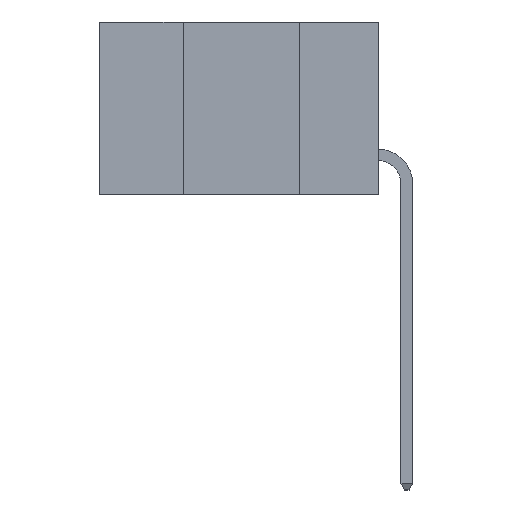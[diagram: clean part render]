
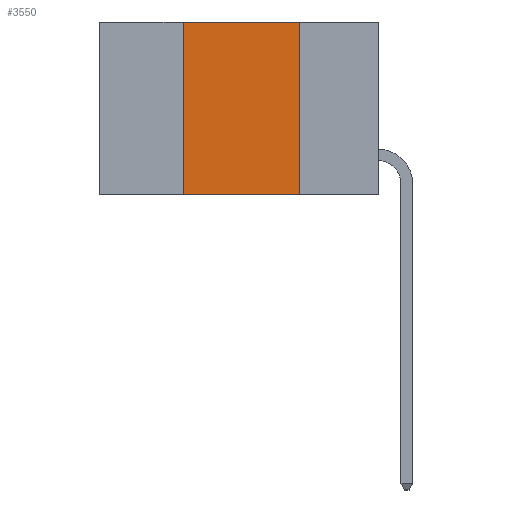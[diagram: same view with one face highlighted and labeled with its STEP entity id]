
A CAD part, left-side view. The second image highlights one B-rep face of the part: STEP entity #3550.
In plain terms, the highlighted planar face has unit normal (-1, 0, 0).
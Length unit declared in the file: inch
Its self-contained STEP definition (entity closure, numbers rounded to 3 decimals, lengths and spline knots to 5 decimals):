
#623 = AXIS2_PLACEMENT_3D ( 'NONE', #3833, #1502, #4617 ) ;
#794 = CARTESIAN_POINT ( 'NONE',  ( 0., 0.42, 0. ) ) ;
#1416 = CARTESIAN_POINT ( 'NONE',  ( 0., 0.6, 0. ) ) ;
#1425 = DIRECTION ( 'NONE',  ( 0., -1., 0. ) ) ;
#1502 = DIRECTION ( 'NONE',  ( 1., 0., 0. ) ) ;
#1968 = ORIENTED_EDGE ( 'NONE', *, *, #6898, .F. ) ;
#2775 = CARTESIAN_POINT ( 'NONE',  ( 0., 0.17, 0. ) ) ;
#2844 = VERTEX_POINT ( 'NONE', #794 ) ;
#3081 = VERTEX_POINT ( 'NONE', #2775 ) ;
#3270 = ORIENTED_EDGE ( 'NONE', *, *, #10433, .T. ) ;
#3459 = LINE ( 'NONE', #7327, #10250 ) ;
#3550 = ADVANCED_FACE ( 'NONE', ( #7556 ), #11281, .F. ) ;
#3833 = CARTESIAN_POINT ( 'NONE',  ( 0., 0.6, 0. ) ) ;
#4165 = EDGE_CURVE ( 'NONE', #3081, #7502, #6405, .T. ) ;
#4617 = DIRECTION ( 'NONE',  ( 0., 0., -1. ) ) ;
#4892 = CARTESIAN_POINT ( 'NONE',  ( 0., 0.6, -0.37 ) ) ;
#5650 = VERTEX_POINT ( 'NONE', #8396 ) ;
#5825 = DIRECTION ( 'NONE',  ( 0., -1., 0. ) ) ;
#5876 = EDGE_CURVE ( 'NONE', #5650, #2844, #3459, .T. ) ;
#6405 = LINE ( 'NONE', #10267, #8492 ) ;
#6553 = EDGE_LOOP ( 'NONE', ( #7065, #1968, #6751, #3270 ) ) ;
#6751 = ORIENTED_EDGE ( 'NONE', *, *, #5876, .F. ) ;
#6898 = EDGE_CURVE ( 'NONE', #2844, #3081, #11330, .T. ) ;
#7065 = ORIENTED_EDGE ( 'NONE', *, *, #4165, .F. ) ;
#7169 = DIRECTION ( 'NONE',  ( 0., 0., 1. ) ) ;
#7327 = CARTESIAN_POINT ( 'NONE',  ( 0., 0.42, -0.37 ) ) ;
#7502 = VERTEX_POINT ( 'NONE', #10383 ) ;
#7556 = FACE_OUTER_BOUND ( 'NONE', #6553, .T. ) ;
#8396 = CARTESIAN_POINT ( 'NONE',  ( 0., 0.42, -0.37 ) ) ;
#8492 = VECTOR ( 'NONE', #8960, 39.37008 ) ;
#8960 = DIRECTION ( 'NONE',  ( 0., 0., -1. ) ) ;
#9430 = VECTOR ( 'NONE', #1425, 39.37008 ) ;
#9753 = VECTOR ( 'NONE', #5825, 39.37008 ) ;
#10014 = LINE ( 'NONE', #4892, #9753 ) ;
#10250 = VECTOR ( 'NONE', #7169, 39.37008 ) ;
#10267 = CARTESIAN_POINT ( 'NONE',  ( 0., 0.17, -0.37 ) ) ;
#10383 = CARTESIAN_POINT ( 'NONE',  ( 0., 0.17, -0.37 ) ) ;
#10433 = EDGE_CURVE ( 'NONE', #5650, #7502, #10014, .T. ) ;
#11281 = PLANE ( 'NONE',  #623 ) ;
#11330 = LINE ( 'NONE', #1416, #9430 ) ;
